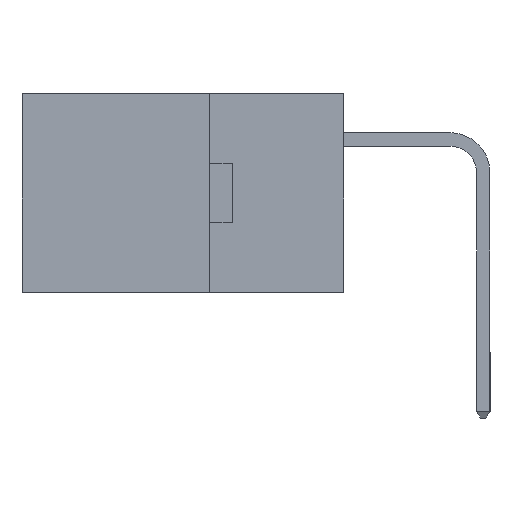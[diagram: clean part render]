
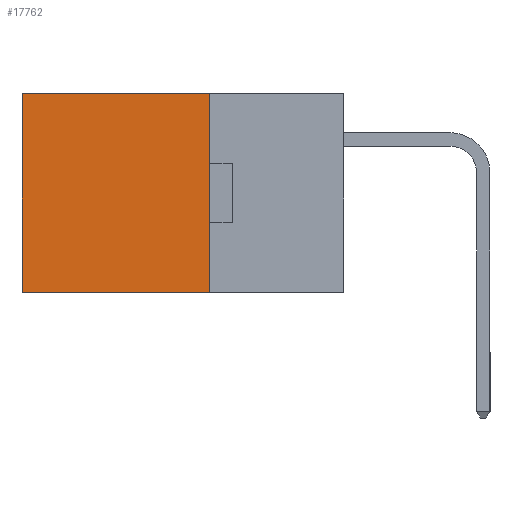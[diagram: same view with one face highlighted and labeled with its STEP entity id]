
A CAD part, left-side view. The second image highlights one B-rep face of the part: STEP entity #17762.
In plain terms, the highlighted planar face has unit normal (-1, 0, 0).
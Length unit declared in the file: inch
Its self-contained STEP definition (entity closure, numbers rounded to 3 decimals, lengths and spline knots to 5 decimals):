
#366 = CARTESIAN_POINT ( 'NONE',  ( 0.2615, 0.6, -0.37 ) ) ;
#3296 = LINE ( 'NONE', #5434, #14197 ) ;
#3684 = VERTEX_POINT ( 'NONE', #4253 ) ;
#4253 = CARTESIAN_POINT ( 'NONE',  ( 0.2615, 0.6, -0.37 ) ) ;
#4332 = EDGE_CURVE ( 'NONE', #16356, #9864, #20833, .T. ) ;
#4595 = LINE ( 'NONE', #4724, #16047 ) ;
#4724 = CARTESIAN_POINT ( 'NONE',  ( 0.2615, 0.25, -0.37 ) ) ;
#4991 = DIRECTION ( 'NONE',  ( 0., 1., 0. ) ) ;
#5434 = CARTESIAN_POINT ( 'NONE',  ( 0.2615, 0.25, -0.37 ) ) ;
#5560 = PLANE ( 'NONE',  #17663 ) ;
#6184 = EDGE_CURVE ( 'NONE', #12221, #3684, #4595, .T. ) ;
#6843 = ORIENTED_EDGE ( 'NONE', *, *, #4332, .T. ) ;
#9306 = CARTESIAN_POINT ( 'NONE',  ( 0.2615, 0.6, 0. ) ) ;
#9320 = DIRECTION ( 'NONE',  ( 0., 0., -1. ) ) ;
#9603 = VECTOR ( 'NONE', #20738, 39.37008 ) ;
#9864 = VERTEX_POINT ( 'NONE', #9306 ) ;
#10925 = ORIENTED_EDGE ( 'NONE', *, *, #19098, .F. ) ;
#11584 = DIRECTION ( 'NONE',  ( 1., 0., 0. ) ) ;
#12221 = VERTEX_POINT ( 'NONE', #17354 ) ;
#12746 = DIRECTION ( 'NONE',  ( 0., 1., 0. ) ) ;
#14197 = VECTOR ( 'NONE', #15458, 39.37008 ) ;
#15400 = ORIENTED_EDGE ( 'NONE', *, *, #6184, .F. ) ;
#15458 = DIRECTION ( 'NONE',  ( 0., 0., -1. ) ) ;
#15459 = CARTESIAN_POINT ( 'NONE',  ( 0.2615, 0.25, -0.37 ) ) ;
#16047 = VECTOR ( 'NONE', #12746, 39.37008 ) ;
#16356 = VERTEX_POINT ( 'NONE', #16523 ) ;
#16523 = CARTESIAN_POINT ( 'NONE',  ( 0.2615, 0.25, 0. ) ) ;
#17354 = CARTESIAN_POINT ( 'NONE',  ( 0.2615, 0.25, -0.37 ) ) ;
#17663 = AXIS2_PLACEMENT_3D ( 'NONE', #15459, #11584, #9320 ) ;
#17762 = ADVANCED_FACE ( 'NONE', ( #23406 ), #5560, .F. ) ;
#17781 = EDGE_LOOP ( 'NONE', ( #19899, #15400, #10925, #6843 ) ) ;
#19098 = EDGE_CURVE ( 'NONE', #16356, #12221, #3296, .T. ) ;
#19899 = ORIENTED_EDGE ( 'NONE', *, *, #22165, .T. ) ;
#20272 = VECTOR ( 'NONE', #4991, 39.37008 ) ;
#20738 = DIRECTION ( 'NONE',  ( 0., 0., -1. ) ) ;
#20833 = LINE ( 'NONE', #21605, #20272 ) ;
#21605 = CARTESIAN_POINT ( 'NONE',  ( 0.2615, 0.25, 0. ) ) ;
#22165 = EDGE_CURVE ( 'NONE', #9864, #3684, #22754, .T. ) ;
#22754 = LINE ( 'NONE', #366, #9603 ) ;
#23406 = FACE_OUTER_BOUND ( 'NONE', #17781, .T. ) ;
